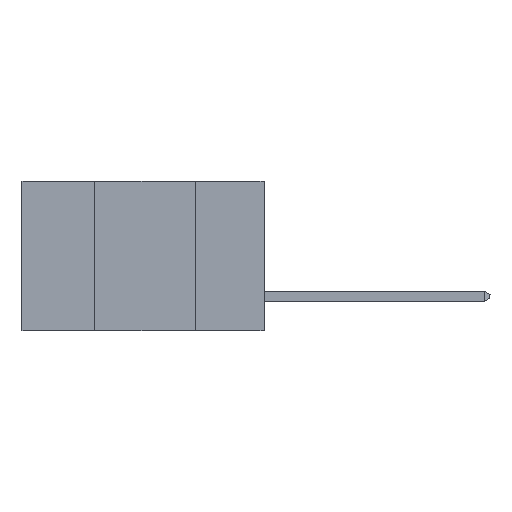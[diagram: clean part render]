
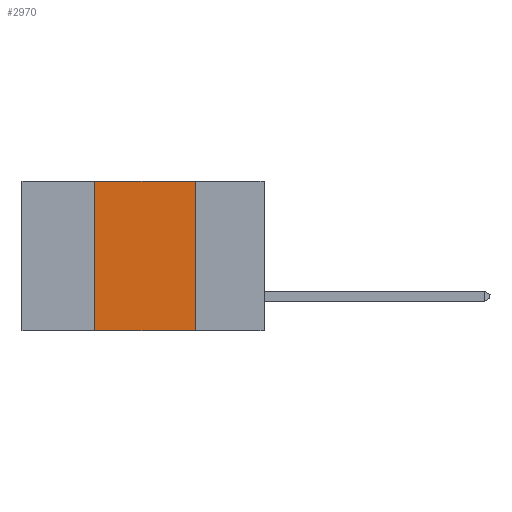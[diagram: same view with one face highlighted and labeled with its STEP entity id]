
A CAD part, left-side view. The second image highlights one B-rep face of the part: STEP entity #2970.
In plain terms, the highlighted planar face has unit normal (-1, 0, 0).
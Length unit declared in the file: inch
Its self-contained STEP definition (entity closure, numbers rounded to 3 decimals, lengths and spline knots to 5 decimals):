
#322 = VECTOR ( 'NONE', #5191, 39.37008 ) ;
#673 = DIRECTION ( 'NONE',  ( 0., 0., -1. ) ) ;
#1626 = VECTOR ( 'NONE', #2267, 39.37008 ) ;
#1884 = EDGE_LOOP ( 'NONE', ( #8468, #5463, #7922, #11265 ) ) ;
#1988 = VERTEX_POINT ( 'NONE', #6109 ) ;
#2267 = DIRECTION ( 'NONE',  ( 0., 0., -1. ) ) ;
#2401 = AXIS2_PLACEMENT_3D ( 'NONE', #5346, #14177, #673 ) ;
#2970 = ADVANCED_FACE ( 'NONE', ( #2999 ), #6489, .F. ) ;
#2999 = FACE_OUTER_BOUND ( 'NONE', #1884, .T. ) ;
#3152 = LINE ( 'NONE', #11487, #5703 ) ;
#3227 = LINE ( 'NONE', #4154, #322 ) ;
#3289 = EDGE_CURVE ( 'NONE', #9383, #9427, #3152, .T. ) ;
#4154 = CARTESIAN_POINT ( 'NONE',  ( 0., 0.6, 0. ) ) ;
#4233 = EDGE_CURVE ( 'NONE', #1988, #9427, #7286, .T. ) ;
#4952 = DIRECTION ( 'NONE',  ( 0., -1., 0. ) ) ;
#5191 = DIRECTION ( 'NONE',  ( 0., -1., 0. ) ) ;
#5346 = CARTESIAN_POINT ( 'NONE',  ( 0., 0.6, 0. ) ) ;
#5463 = ORIENTED_EDGE ( 'NONE', *, *, #13193, .F. ) ;
#5703 = VECTOR ( 'NONE', #4952, 39.37008 ) ;
#5752 = CARTESIAN_POINT ( 'NONE',  ( 0., 0.42, -0.37 ) ) ;
#6062 = CARTESIAN_POINT ( 'NONE',  ( 0., 0.42, 0. ) ) ;
#6109 = CARTESIAN_POINT ( 'NONE',  ( 0., 0.17, 0. ) ) ;
#6489 = PLANE ( 'NONE',  #2401 ) ;
#6635 = EDGE_CURVE ( 'NONE', #9383, #6838, #8775, .T. ) ;
#6838 = VERTEX_POINT ( 'NONE', #6062 ) ;
#7286 = LINE ( 'NONE', #10966, #1626 ) ;
#7745 = VECTOR ( 'NONE', #14133, 39.37008 ) ;
#7922 = ORIENTED_EDGE ( 'NONE', *, *, #6635, .F. ) ;
#8468 = ORIENTED_EDGE ( 'NONE', *, *, #4233, .F. ) ;
#8775 = LINE ( 'NONE', #12999, #7745 ) ;
#9383 = VERTEX_POINT ( 'NONE', #5752 ) ;
#9427 = VERTEX_POINT ( 'NONE', #13282 ) ;
#10966 = CARTESIAN_POINT ( 'NONE',  ( 0., 0.17, 0. ) ) ;
#11265 = ORIENTED_EDGE ( 'NONE', *, *, #3289, .T. ) ;
#11487 = CARTESIAN_POINT ( 'NONE',  ( 0., 0.6, -0.37 ) ) ;
#12999 = CARTESIAN_POINT ( 'NONE',  ( 0., 0.42, 0. ) ) ;
#13193 = EDGE_CURVE ( 'NONE', #6838, #1988, #3227, .T. ) ;
#13282 = CARTESIAN_POINT ( 'NONE',  ( 0., 0.17, -0.37 ) ) ;
#14133 = DIRECTION ( 'NONE',  ( 0., 0., 1. ) ) ;
#14177 = DIRECTION ( 'NONE',  ( 1., 0., 0. ) ) ;
